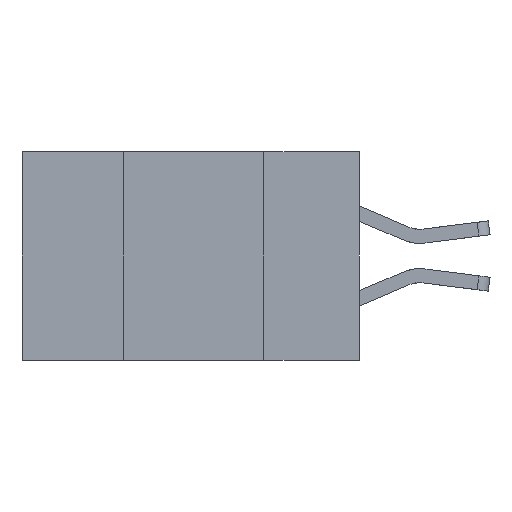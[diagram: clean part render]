
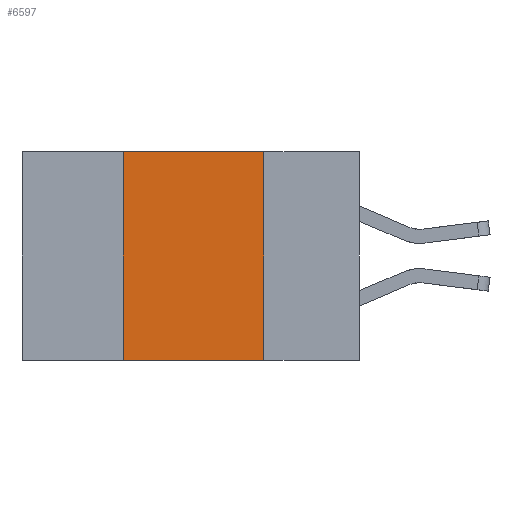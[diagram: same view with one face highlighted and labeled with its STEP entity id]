
A CAD part, left-side view. The second image highlights one B-rep face of the part: STEP entity #6597.
In plain terms, the highlighted planar face has unit normal (-1, 0, 0).
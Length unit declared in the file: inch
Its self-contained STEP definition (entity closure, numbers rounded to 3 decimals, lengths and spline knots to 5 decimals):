
#676 = CARTESIAN_POINT ( 'NONE',  ( 0., 0.42, 0. ) ) ;
#837 = VERTEX_POINT ( 'NONE', #8485 ) ;
#1188 = CARTESIAN_POINT ( 'NONE',  ( 0., 0.17, -0.37 ) ) ;
#1202 = CARTESIAN_POINT ( 'NONE',  ( 0., 0.6, -0.37 ) ) ;
#3033 = ORIENTED_EDGE ( 'NONE', *, *, #9717, .F. ) ;
#3690 = DIRECTION ( 'NONE',  ( 1., 0., 0. ) ) ;
#3784 = CARTESIAN_POINT ( 'NONE',  ( 0., 0.6, 0. ) ) ;
#4099 = FACE_OUTER_BOUND ( 'NONE', #10824, .T. ) ;
#5345 = ORIENTED_EDGE ( 'NONE', *, *, #6338, .T. ) ;
#5855 = EDGE_CURVE ( 'NONE', #837, #12028, #5879, .T. ) ;
#5879 = LINE ( 'NONE', #12441, #10836 ) ;
#6338 = EDGE_CURVE ( 'NONE', #837, #9519, #9704, .T. ) ;
#6597 = ADVANCED_FACE ( 'NONE', ( #4099 ), #9902, .F. ) ;
#6884 = CARTESIAN_POINT ( 'NONE',  ( 0., 0.6, 0. ) ) ;
#7304 = CARTESIAN_POINT ( 'NONE',  ( 0., 0.17, 0. ) ) ;
#7569 = EDGE_CURVE ( 'NONE', #12028, #9525, #7963, .T. ) ;
#7691 = CARTESIAN_POINT ( 'NONE',  ( 0., 0.17, 0. ) ) ;
#7963 = LINE ( 'NONE', #6884, #12626 ) ;
#8485 = CARTESIAN_POINT ( 'NONE',  ( 0., 0.42, -0.37 ) ) ;
#8571 = VECTOR ( 'NONE', #9616, 39.37008 ) ;
#8743 = LINE ( 'NONE', #7691, #8571 ) ;
#9382 = VECTOR ( 'NONE', #10372, 39.37008 ) ;
#9467 = DIRECTION ( 'NONE',  ( 0., 0., 1. ) ) ;
#9519 = VERTEX_POINT ( 'NONE', #1188 ) ;
#9525 = VERTEX_POINT ( 'NONE', #7304 ) ;
#9616 = DIRECTION ( 'NONE',  ( 0., 0., -1. ) ) ;
#9704 = LINE ( 'NONE', #1202, #9382 ) ;
#9717 = EDGE_CURVE ( 'NONE', #9525, #9519, #8743, .T. ) ;
#9902 = PLANE ( 'NONE',  #12543 ) ;
#10372 = DIRECTION ( 'NONE',  ( 0., -1., 0. ) ) ;
#10824 = EDGE_LOOP ( 'NONE', ( #3033, #12396, #13123, #5345 ) ) ;
#10836 = VECTOR ( 'NONE', #9467, 39.37008 ) ;
#12028 = VERTEX_POINT ( 'NONE', #676 ) ;
#12396 = ORIENTED_EDGE ( 'NONE', *, *, #7569, .F. ) ;
#12441 = CARTESIAN_POINT ( 'NONE',  ( 0., 0.42, 0. ) ) ;
#12543 = AXIS2_PLACEMENT_3D ( 'NONE', #3784, #3690, #12917 ) ;
#12626 = VECTOR ( 'NONE', #12916, 39.37008 ) ;
#12916 = DIRECTION ( 'NONE',  ( 0., -1., 0. ) ) ;
#12917 = DIRECTION ( 'NONE',  ( 0., 0., -1. ) ) ;
#13123 = ORIENTED_EDGE ( 'NONE', *, *, #5855, .F. ) ;
